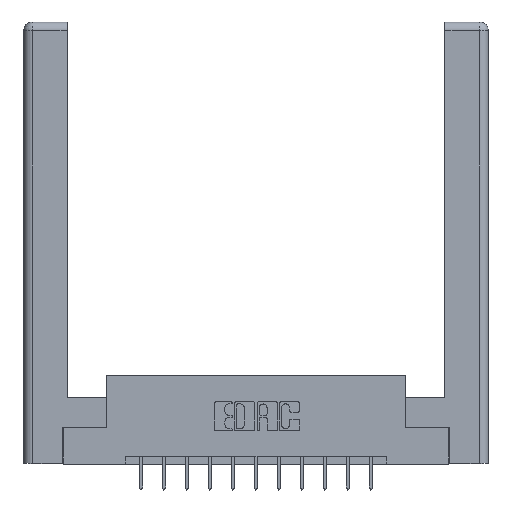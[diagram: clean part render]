
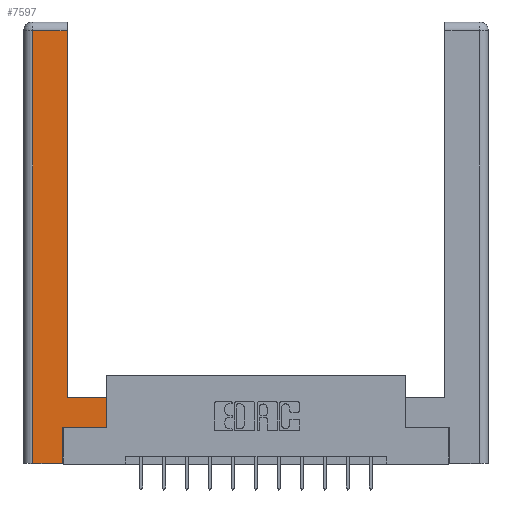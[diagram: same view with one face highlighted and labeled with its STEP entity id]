
A CAD part, top view. The second image highlights one B-rep face of the part: STEP entity #7597.
In plain terms, the highlighted planar face has unit normal (0, 0, 1).
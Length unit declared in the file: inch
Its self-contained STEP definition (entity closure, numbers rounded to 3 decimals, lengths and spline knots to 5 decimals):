
#176 = ORIENTED_EDGE ( 'NONE', *, *, #8775, .T. ) ;
#284 = DIRECTION ( 'NONE',  ( -1., 0., 0. ) ) ;
#328 = ORIENTED_EDGE ( 'NONE', *, *, #1191, .T. ) ;
#615 = ORIENTED_EDGE ( 'NONE', *, *, #7715, .T. ) ;
#952 = VERTEX_POINT ( 'NONE', #3817 ) ;
#1016 = PLANE ( 'NONE',  #2006 ) ;
#1067 = DIRECTION ( 'NONE',  ( -1., 0., 0. ) ) ;
#1105 = ORIENTED_EDGE ( 'NONE', *, *, #11545, .T. ) ;
#1120 = DIRECTION ( 'NONE',  ( -1., 0., 0. ) ) ;
#1191 = EDGE_CURVE ( 'NONE', #3660, #12236, #7397, .T. ) ;
#1376 = DIRECTION ( 'NONE',  ( 1., 0., 0. ) ) ;
#1417 = CARTESIAN_POINT ( 'NONE',  ( 0.265, 0.245, 0. ) ) ;
#1455 = CARTESIAN_POINT ( 'NONE',  ( 0.565, 0.45, 0. ) ) ;
#1948 = CARTESIAN_POINT ( 'NONE',  ( 0.565, 0.245, 0. ) ) ;
#2006 = AXIS2_PLACEMENT_3D ( 'NONE', #13900, #10386, #1120 ) ;
#2425 = LINE ( 'NONE', #13276, #7043 ) ;
#2502 = CARTESIAN_POINT ( 'NONE',  ( 0.565, 0.245, 0. ) ) ;
#2566 = VECTOR ( 'NONE', #5944, 39.37008 ) ;
#2765 = CARTESIAN_POINT ( 'NONE',  ( 0.295, 2.94, 0. ) ) ;
#2983 = CARTESIAN_POINT ( 'NONE',  ( 0.265, 0., 0. ) ) ;
#3646 = CARTESIAN_POINT ( 'NONE',  ( 0.565, 0.45, 0. ) ) ;
#3660 = VERTEX_POINT ( 'NONE', #5757 ) ;
#3817 = CARTESIAN_POINT ( 'NONE',  ( 0.0615, 0., 0. ) ) ;
#4472 = VECTOR ( 'NONE', #8514, 39.37008 ) ;
#4592 = LINE ( 'NONE', #13312, #7164 ) ;
#4870 = EDGE_LOOP ( 'NONE', ( #176, #7060, #15187, #7083, #328, #1105, #8341, #615 ) ) ;
#5203 = VERTEX_POINT ( 'NONE', #3646 ) ;
#5270 = CARTESIAN_POINT ( 'NONE',  ( 0.295, 0.45, 0. ) ) ;
#5563 = EDGE_CURVE ( 'NONE', #7866, #5992, #9259, .T. ) ;
#5757 = CARTESIAN_POINT ( 'NONE',  ( 0.265, 0., 0. ) ) ;
#5944 = DIRECTION ( 'NONE',  ( 0., -1., 0. ) ) ;
#5992 = VERTEX_POINT ( 'NONE', #6542 ) ;
#6029 = EDGE_CURVE ( 'NONE', #952, #3660, #9244, .T. ) ;
#6542 = CARTESIAN_POINT ( 'NONE',  ( 0.0615, 2.94, 0. ) ) ;
#7043 = VECTOR ( 'NONE', #13176, 39.37008 ) ;
#7060 = ORIENTED_EDGE ( 'NONE', *, *, #5563, .T. ) ;
#7083 = ORIENTED_EDGE ( 'NONE', *, *, #6029, .T. ) ;
#7164 = VECTOR ( 'NONE', #284, 39.37008 ) ;
#7242 = EDGE_CURVE ( 'NONE', #5992, #952, #14357, .T. ) ;
#7397 = LINE ( 'NONE', #1417, #4472 ) ;
#7597 = ADVANCED_FACE ( 'NONE', ( #10675 ), #1016, .F. ) ;
#7715 = EDGE_CURVE ( 'NONE', #5203, #11154, #4592, .T. ) ;
#7826 = DIRECTION ( 'NONE',  ( 1., 0., 0. ) ) ;
#7866 = VERTEX_POINT ( 'NONE', #2765 ) ;
#8341 = ORIENTED_EDGE ( 'NONE', *, *, #10954, .T. ) ;
#8514 = DIRECTION ( 'NONE',  ( 0., 1., 0. ) ) ;
#8775 = EDGE_CURVE ( 'NONE', #11154, #7866, #2425, .T. ) ;
#8915 = VECTOR ( 'NONE', #1067, 39.37008 ) ;
#9244 = LINE ( 'NONE', #2983, #11639 ) ;
#9259 = LINE ( 'NONE', #15264, #8915 ) ;
#9584 = VECTOR ( 'NONE', #9638, 39.37008 ) ;
#9638 = DIRECTION ( 'NONE',  ( 0., 1., 0. ) ) ;
#10107 = LINE ( 'NONE', #2502, #12876 ) ;
#10386 = DIRECTION ( 'NONE',  ( 0., 0., -1. ) ) ;
#10675 = FACE_OUTER_BOUND ( 'NONE', #4870, .T. ) ;
#10711 = CARTESIAN_POINT ( 'NONE',  ( 0.0615, 0., 0. ) ) ;
#10886 = CARTESIAN_POINT ( 'NONE',  ( 0.265, 0.245, 0. ) ) ;
#10954 = EDGE_CURVE ( 'NONE', #14985, #5203, #13828, .T. ) ;
#11154 = VERTEX_POINT ( 'NONE', #5270 ) ;
#11545 = EDGE_CURVE ( 'NONE', #12236, #14985, #10107, .T. ) ;
#11639 = VECTOR ( 'NONE', #7826, 39.37008 ) ;
#12236 = VERTEX_POINT ( 'NONE', #10886 ) ;
#12876 = VECTOR ( 'NONE', #1376, 39.37008 ) ;
#13176 = DIRECTION ( 'NONE',  ( 0., 1., 0. ) ) ;
#13276 = CARTESIAN_POINT ( 'NONE',  ( 0.295, 3., 0. ) ) ;
#13312 = CARTESIAN_POINT ( 'NONE',  ( 0.295, 0.45, 0. ) ) ;
#13828 = LINE ( 'NONE', #1455, #9584 ) ;
#13900 = CARTESIAN_POINT ( 'NONE',  ( 0., 0., 0. ) ) ;
#14357 = LINE ( 'NONE', #10711, #2566 ) ;
#14985 = VERTEX_POINT ( 'NONE', #1948 ) ;
#15187 = ORIENTED_EDGE ( 'NONE', *, *, #7242, .T. ) ;
#15264 = CARTESIAN_POINT ( 'NONE',  ( 0.0615, 2.94, 0. ) ) ;
